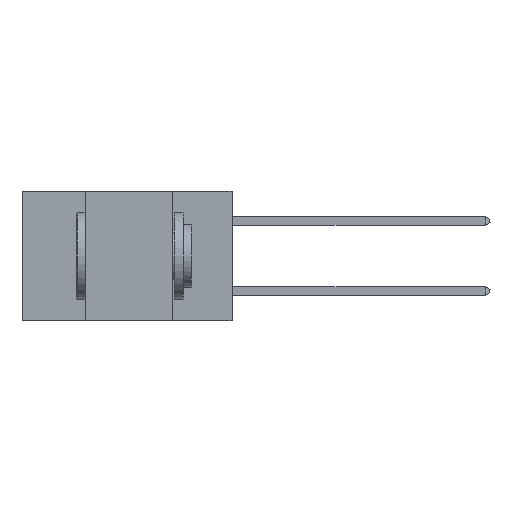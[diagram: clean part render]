
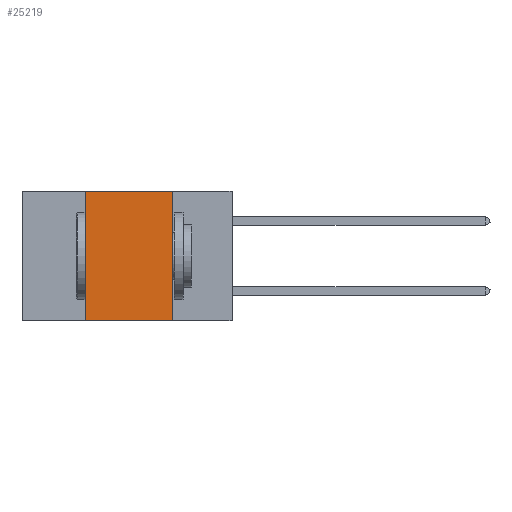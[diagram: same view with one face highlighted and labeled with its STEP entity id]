
A CAD part, left-side view. The second image highlights one B-rep face of the part: STEP entity #25219.
In plain terms, the highlighted planar face has unit normal (-1, 0, 0).
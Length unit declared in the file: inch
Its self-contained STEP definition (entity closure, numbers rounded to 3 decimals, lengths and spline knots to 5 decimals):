
#436 = EDGE_LOOP ( 'NONE', ( #19230, #21167, #37367, #30358 ) ) ;
#1706 = PLANE ( 'NONE',  #31278 ) ;
#2018 = VECTOR ( 'NONE', #9255, 39.37008 ) ;
#3062 = VECTOR ( 'NONE', #22427, 39.37008 ) ;
#3981 = LINE ( 'NONE', #6071, #2018 ) ;
#4598 = EDGE_CURVE ( 'NONE', #34992, #25554, #11457, .T. ) ;
#4877 = CARTESIAN_POINT ( 'NONE',  ( 0., 0.6, 0. ) ) ;
#5503 = VERTEX_POINT ( 'NONE', #19007 ) ;
#5531 = CARTESIAN_POINT ( 'NONE',  ( 0., 0.42, 0. ) ) ;
#6071 = CARTESIAN_POINT ( 'NONE',  ( 0., 0.6, 0. ) ) ;
#6702 = LINE ( 'NONE', #11360, #14073 ) ;
#8071 = DIRECTION ( 'NONE',  ( 1., 0., 0. ) ) ;
#8730 = DIRECTION ( 'NONE',  ( 0., 0., 1. ) ) ;
#9255 = DIRECTION ( 'NONE',  ( 0., -1., 0. ) ) ;
#11360 = CARTESIAN_POINT ( 'NONE',  ( 0., 0.17, 0. ) ) ;
#11457 = LINE ( 'NONE', #19327, #3062 ) ;
#14073 = VECTOR ( 'NONE', #23603, 39.37008 ) ;
#16530 = VERTEX_POINT ( 'NONE', #28536 ) ;
#17956 = EDGE_CURVE ( 'NONE', #34992, #5503, #24947, .T. ) ;
#19007 = CARTESIAN_POINT ( 'NONE',  ( 0., 0.42, 0. ) ) ;
#19230 = ORIENTED_EDGE ( 'NONE', *, *, #39138, .F. ) ;
#19327 = CARTESIAN_POINT ( 'NONE',  ( 0., 0.6, -0.37 ) ) ;
#21167 = ORIENTED_EDGE ( 'NONE', *, *, #22225, .F. ) ;
#22225 = EDGE_CURVE ( 'NONE', #5503, #16530, #3981, .T. ) ;
#22427 = DIRECTION ( 'NONE',  ( 0., -1., 0. ) ) ;
#23603 = DIRECTION ( 'NONE',  ( 0., 0., -1. ) ) ;
#24947 = LINE ( 'NONE', #5531, #39120 ) ;
#25219 = ADVANCED_FACE ( 'NONE', ( #37705 ), #1706, .F. ) ;
#25554 = VERTEX_POINT ( 'NONE', #37704 ) ;
#28536 = CARTESIAN_POINT ( 'NONE',  ( 0., 0.17, 0. ) ) ;
#29870 = DIRECTION ( 'NONE',  ( 0., 0., -1. ) ) ;
#29976 = CARTESIAN_POINT ( 'NONE',  ( 0., 0.42, -0.37 ) ) ;
#30358 = ORIENTED_EDGE ( 'NONE', *, *, #4598, .T. ) ;
#31278 = AXIS2_PLACEMENT_3D ( 'NONE', #4877, #8071, #29870 ) ;
#34992 = VERTEX_POINT ( 'NONE', #29976 ) ;
#37367 = ORIENTED_EDGE ( 'NONE', *, *, #17956, .F. ) ;
#37705 = FACE_OUTER_BOUND ( 'NONE', #436, .T. ) ;
#37704 = CARTESIAN_POINT ( 'NONE',  ( 0., 0.17, -0.37 ) ) ;
#39120 = VECTOR ( 'NONE', #8730, 39.37008 ) ;
#39138 = EDGE_CURVE ( 'NONE', #16530, #25554, #6702, .T. ) ;
